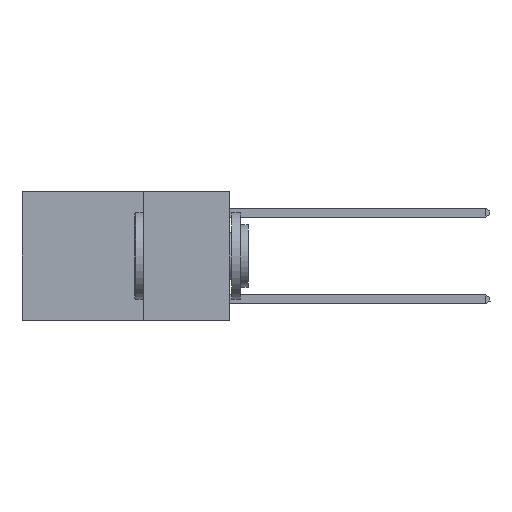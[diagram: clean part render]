
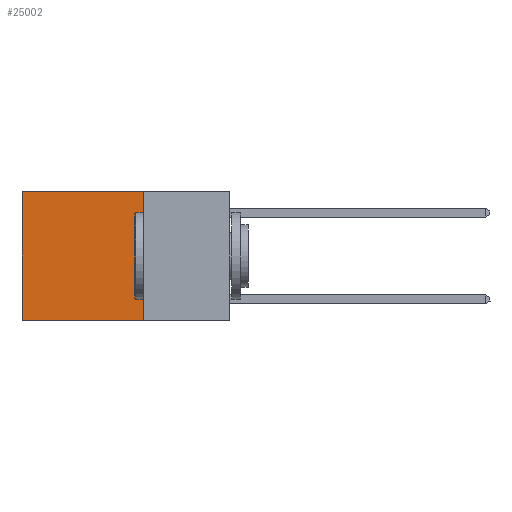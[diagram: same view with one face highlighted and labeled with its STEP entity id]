
A CAD part, left-side view. The second image highlights one B-rep face of the part: STEP entity #25002.
In plain terms, the highlighted planar face has unit normal (-1, 0, 0).
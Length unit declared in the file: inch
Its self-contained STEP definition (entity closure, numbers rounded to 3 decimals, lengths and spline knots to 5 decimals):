
#161 = EDGE_CURVE ( 'NONE', #1435, #23618, #7265, .T. ) ;
#514 = ORIENTED_EDGE ( 'NONE', *, *, #8227, .T. ) ;
#1435 = VERTEX_POINT ( 'NONE', #27863 ) ;
#1665 = CARTESIAN_POINT ( 'NONE',  ( 0.2625, 0.25, -0.37 ) ) ;
#1824 = VECTOR ( 'NONE', #21607, 39.37008 ) ;
#5383 = CARTESIAN_POINT ( 'NONE',  ( 0.2625, 0.6, 0. ) ) ;
#7223 = AXIS2_PLACEMENT_3D ( 'NONE', #13528, #30968, #16038 ) ;
#7265 = LINE ( 'NONE', #30334, #27126 ) ;
#8227 = EDGE_CURVE ( 'NONE', #1435, #30581, #24654, .T. ) ;
#9258 = LINE ( 'NONE', #1665, #1824 ) ;
#11774 = EDGE_LOOP ( 'NONE', ( #13903, #12064, #25298, #514 ) ) ;
#12002 = EDGE_CURVE ( 'NONE', #23618, #18728, #9258, .T. ) ;
#12064 = ORIENTED_EDGE ( 'NONE', *, *, #12002, .F. ) ;
#12123 = DIRECTION ( 'NONE',  ( 0., 1., 0. ) ) ;
#12322 = EDGE_CURVE ( 'NONE', #30581, #18728, #31423, .T. ) ;
#12879 = DIRECTION ( 'NONE',  ( 0., 0., -1. ) ) ;
#13528 = CARTESIAN_POINT ( 'NONE',  ( 0.2625, 0.25, 0. ) ) ;
#13903 = ORIENTED_EDGE ( 'NONE', *, *, #12322, .T. ) ;
#16038 = DIRECTION ( 'NONE',  ( 0., 0., -1. ) ) ;
#18185 = VECTOR ( 'NONE', #27824, 39.37008 ) ;
#18728 = VERTEX_POINT ( 'NONE', #20704 ) ;
#20704 = CARTESIAN_POINT ( 'NONE',  ( 0.2625, 0.6, -0.37 ) ) ;
#21607 = DIRECTION ( 'NONE',  ( 0., 1., 0. ) ) ;
#22020 = CARTESIAN_POINT ( 'NONE',  ( 0.2625, 0.25, 0. ) ) ;
#23618 = VERTEX_POINT ( 'NONE', #31143 ) ;
#24654 = LINE ( 'NONE', #22020, #29725 ) ;
#24934 = FACE_OUTER_BOUND ( 'NONE', #11774, .T. ) ;
#25002 = ADVANCED_FACE ( 'NONE', ( #24934 ), #25949, .F. ) ;
#25298 = ORIENTED_EDGE ( 'NONE', *, *, #161, .F. ) ;
#25949 = PLANE ( 'NONE',  #7223 ) ;
#27126 = VECTOR ( 'NONE', #12879, 39.37008 ) ;
#27824 = DIRECTION ( 'NONE',  ( 0., 0., -1. ) ) ;
#27863 = CARTESIAN_POINT ( 'NONE',  ( 0.2625, 0.25, 0. ) ) ;
#28009 = CARTESIAN_POINT ( 'NONE',  ( 0.2625, 0.6, 0. ) ) ;
#29725 = VECTOR ( 'NONE', #12123, 39.37008 ) ;
#30334 = CARTESIAN_POINT ( 'NONE',  ( 0.2625, 0.25, 0. ) ) ;
#30581 = VERTEX_POINT ( 'NONE', #28009 ) ;
#30968 = DIRECTION ( 'NONE',  ( 1., 0., 0. ) ) ;
#31143 = CARTESIAN_POINT ( 'NONE',  ( 0.2625, 0.25, -0.37 ) ) ;
#31423 = LINE ( 'NONE', #5383, #18185 ) ;
